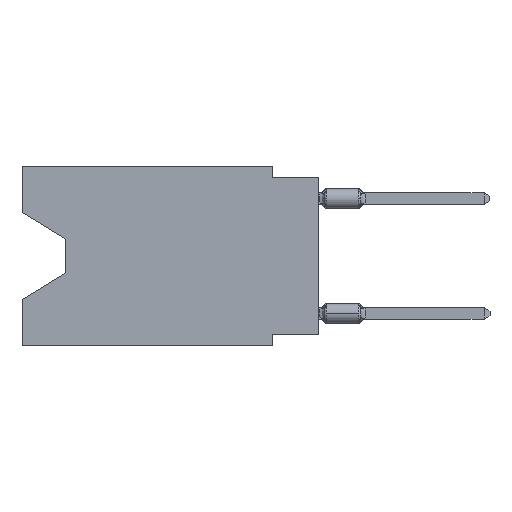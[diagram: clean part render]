
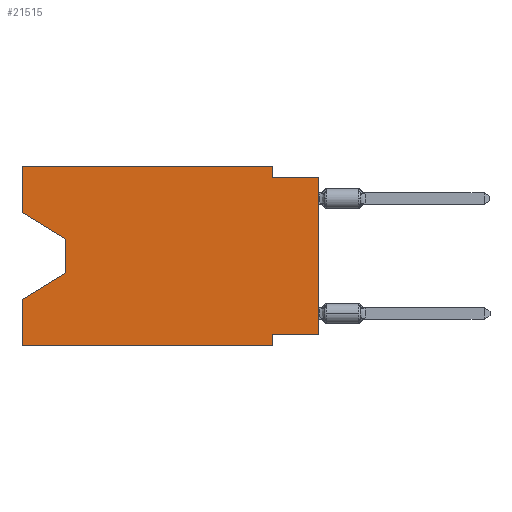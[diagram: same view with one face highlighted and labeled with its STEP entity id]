
A CAD part, left-side view. The second image highlights one B-rep face of the part: STEP entity #21515.
In plain terms, the highlighted planar face has unit normal (-1, 0, 0).
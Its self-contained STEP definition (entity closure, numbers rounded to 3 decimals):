
#247 = PLANE ( 'NONE',  #7075 ) ;
#301 = VERTEX_POINT ( 'NONE', #19741 ) ;
#318 = CARTESIAN_POINT ( 'NONE',  ( 0., 16.383, -2.546 ) ) ;
#610 = CARTESIAN_POINT ( 'NONE',  ( 0., 16.383, 0. ) ) ;
#723 = CARTESIAN_POINT ( 'NONE',  ( 0., 16.383, -2.546 ) ) ;
#751 = DIRECTION ( 'NONE',  ( 0., 0., -1. ) ) ;
#996 = CARTESIAN_POINT ( 'NONE',  ( 0., 2.54, 0. ) ) ;
#1258 = ORIENTED_EDGE ( 'NONE', *, *, #8355, .F. ) ;
#1450 = EDGE_LOOP ( 'NONE', ( #6111, #10877, #15848, #10048, #2695, #10234, #1258, #2881, #22175, #19220, #5291, #13196 ) ) ;
#1513 = VERTEX_POINT ( 'NONE', #18619 ) ;
#1657 = DIRECTION ( 'NONE',  ( 0., 0., 1. ) ) ;
#2146 = CARTESIAN_POINT ( 'NONE',  ( 0., 13.97, -5.893 ) ) ;
#2314 = FACE_OUTER_BOUND ( 'NONE', #1450, .T. ) ;
#2417 = VECTOR ( 'NONE', #21864, 1000. ) ;
#2502 = EDGE_CURVE ( 'NONE', #1513, #17818, #13295, .T. ) ;
#2695 = ORIENTED_EDGE ( 'NONE', *, *, #2502, .T. ) ;
#2749 = VERTEX_POINT ( 'NONE', #3464 ) ;
#2881 = ORIENTED_EDGE ( 'NONE', *, *, #21891, .T. ) ;
#3350 = DIRECTION ( 'NONE',  ( 0., 0.855, -0.519 ) ) ;
#3464 = CARTESIAN_POINT ( 'NONE',  ( 0., 16.383, -7.36 ) ) ;
#3947 = EDGE_CURVE ( 'NONE', #13016, #22569, #23340, .T. ) ;
#4218 = CARTESIAN_POINT ( 'NONE',  ( 0., 16.383, -9.906 ) ) ;
#5291 = ORIENTED_EDGE ( 'NONE', *, *, #3947, .F. ) ;
#5308 = LINE ( 'NONE', #8992, #8228 ) ;
#5806 = DIRECTION ( 'NONE',  ( 0., -0.855, -0.519 ) ) ;
#6111 = ORIENTED_EDGE ( 'NONE', *, *, #11681, .T. ) ;
#6910 = LINE ( 'NONE', #14421, #2417 ) ;
#7075 = AXIS2_PLACEMENT_3D ( 'NONE', #610, #17392, #17142 ) ;
#7463 = VECTOR ( 'NONE', #1657, 1000. ) ;
#7479 = VECTOR ( 'NONE', #16758, 1000. ) ;
#7867 = VECTOR ( 'NONE', #751, 1000. ) ;
#8108 = VECTOR ( 'NONE', #22959, 1000. ) ;
#8228 = VECTOR ( 'NONE', #3350, 1000. ) ;
#8355 = EDGE_CURVE ( 'NONE', #10129, #12651, #16994, .T. ) ;
#8411 = CARTESIAN_POINT ( 'NONE',  ( 0., 16.383, 0. ) ) ;
#8992 = CARTESIAN_POINT ( 'NONE',  ( 0., 13.97, -5.893 ) ) ;
#9473 = CARTESIAN_POINT ( 'NONE',  ( 0., 0., -0.635 ) ) ;
#10048 = ORIENTED_EDGE ( 'NONE', *, *, #11553, .F. ) ;
#10129 = VERTEX_POINT ( 'NONE', #23211 ) ;
#10234 = ORIENTED_EDGE ( 'NONE', *, *, #12972, .F. ) ;
#10877 = ORIENTED_EDGE ( 'NONE', *, *, #22303, .T. ) ;
#11553 = EDGE_CURVE ( 'NONE', #1513, #2749, #24061, .T. ) ;
#11681 = EDGE_CURVE ( 'NONE', #20529, #23395, #16973, .T. ) ;
#11979 = LINE ( 'NONE', #8411, #22557 ) ;
#12398 = LINE ( 'NONE', #23148, #23557 ) ;
#12651 = VERTEX_POINT ( 'NONE', #23565 ) ;
#12799 = VECTOR ( 'NONE', #15329, 1000. ) ;
#12972 = EDGE_CURVE ( 'NONE', #12651, #17818, #12398, .T. ) ;
#13016 = VERTEX_POINT ( 'NONE', #16198 ) ;
#13196 = ORIENTED_EDGE ( 'NONE', *, *, #23306, .F. ) ;
#13295 = LINE ( 'NONE', #4218, #15487 ) ;
#13768 = VECTOR ( 'NONE', #5806, 1000. ) ;
#13815 = DIRECTION ( 'NONE',  ( 0., 0., 1. ) ) ;
#14117 = CARTESIAN_POINT ( 'NONE',  ( 0., 2.54, 0. ) ) ;
#14353 = EDGE_CURVE ( 'NONE', #301, #18878, #15231, .T. ) ;
#14421 = CARTESIAN_POINT ( 'NONE',  ( 0., 13.97, -4.013 ) ) ;
#14572 = CARTESIAN_POINT ( 'NONE',  ( 0., 0., 0. ) ) ;
#14870 = VECTOR ( 'NONE', #20498, 1000. ) ;
#15231 = LINE ( 'NONE', #9473, #14870 ) ;
#15329 = DIRECTION ( 'NONE',  ( 0., -1., 0. ) ) ;
#15462 = EDGE_CURVE ( 'NONE', #16036, #2749, #5308, .T. ) ;
#15487 = VECTOR ( 'NONE', #17323, 1000. ) ;
#15848 = ORIENTED_EDGE ( 'NONE', *, *, #15462, .T. ) ;
#16036 = VERTEX_POINT ( 'NONE', #2146 ) ;
#16198 = CARTESIAN_POINT ( 'NONE',  ( 0., 16.383, 0. ) ) ;
#16758 = DIRECTION ( 'NONE',  ( 0., 0., 1. ) ) ;
#16973 = LINE ( 'NONE', #318, #13768 ) ;
#16994 = LINE ( 'NONE', #22841, #8108 ) ;
#17142 = DIRECTION ( 'NONE',  ( 0., 0., -1. ) ) ;
#17323 = DIRECTION ( 'NONE',  ( 0., -1., 0. ) ) ;
#17392 = DIRECTION ( 'NONE',  ( 1., 0., 0. ) ) ;
#17600 = CARTESIAN_POINT ( 'NONE',  ( 0., 13.97, -4.013 ) ) ;
#17807 = CARTESIAN_POINT ( 'NONE',  ( 0., 0., -0.635 ) ) ;
#17818 = VERTEX_POINT ( 'NONE', #18289 ) ;
#18289 = CARTESIAN_POINT ( 'NONE',  ( 0., 2.54, -9.906 ) ) ;
#18619 = CARTESIAN_POINT ( 'NONE',  ( 0., 16.383, -9.906 ) ) ;
#18754 = CARTESIAN_POINT ( 'NONE',  ( 0., 16.383, 0. ) ) ;
#18878 = VERTEX_POINT ( 'NONE', #17807 ) ;
#19220 = ORIENTED_EDGE ( 'NONE', *, *, #20140, .F. ) ;
#19741 = CARTESIAN_POINT ( 'NONE',  ( 0., 2.54, -0.635 ) ) ;
#20140 = EDGE_CURVE ( 'NONE', #22569, #301, #21683, .T. ) ;
#20198 = LINE ( 'NONE', #14572, #7479 ) ;
#20498 = DIRECTION ( 'NONE',  ( 0., -1., 0. ) ) ;
#20529 = VERTEX_POINT ( 'NONE', #723 ) ;
#21515 = ADVANCED_FACE ( 'NONE', ( #2314 ), #247, .F. ) ;
#21683 = LINE ( 'NONE', #14117, #7867 ) ;
#21864 = DIRECTION ( 'NONE',  ( 0., 0., -1. ) ) ;
#21891 = EDGE_CURVE ( 'NONE', #10129, #18878, #20198, .T. ) ;
#22175 = ORIENTED_EDGE ( 'NONE', *, *, #14353, .F. ) ;
#22303 = EDGE_CURVE ( 'NONE', #23395, #16036, #6910, .T. ) ;
#22557 = VECTOR ( 'NONE', #13815, 1000. ) ;
#22569 = VERTEX_POINT ( 'NONE', #996 ) ;
#22582 = CARTESIAN_POINT ( 'NONE',  ( 0., 16.383, 0. ) ) ;
#22841 = CARTESIAN_POINT ( 'NONE',  ( 0., 0., -9.271 ) ) ;
#22959 = DIRECTION ( 'NONE',  ( 0., 1., 0. ) ) ;
#23148 = CARTESIAN_POINT ( 'NONE',  ( 0., 2.54, -9.906 ) ) ;
#23211 = CARTESIAN_POINT ( 'NONE',  ( 0., 0., -9.271 ) ) ;
#23306 = EDGE_CURVE ( 'NONE', #20529, #13016, #11979, .T. ) ;
#23340 = LINE ( 'NONE', #18754, #12799 ) ;
#23395 = VERTEX_POINT ( 'NONE', #17600 ) ;
#23515 = DIRECTION ( 'NONE',  ( 0., 0., -1. ) ) ;
#23557 = VECTOR ( 'NONE', #23515, 1000. ) ;
#23565 = CARTESIAN_POINT ( 'NONE',  ( 0., 2.54, -9.271 ) ) ;
#24061 = LINE ( 'NONE', #22582, #7463 ) ;
